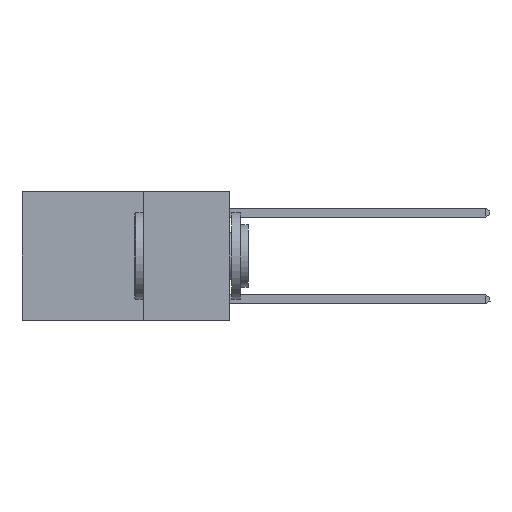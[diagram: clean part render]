
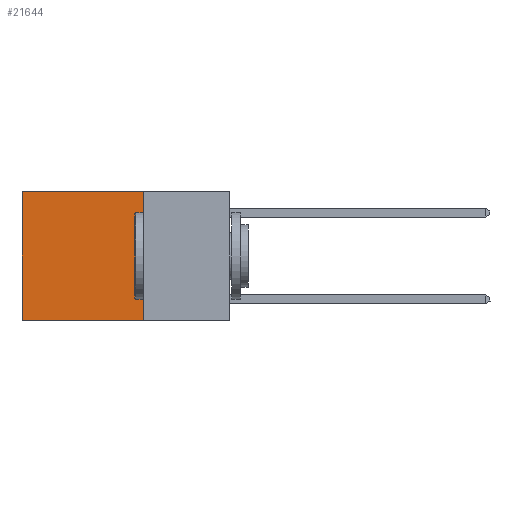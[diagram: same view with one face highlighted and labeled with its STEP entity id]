
A CAD part, left-side view. The second image highlights one B-rep face of the part: STEP entity #21644.
In plain terms, the highlighted planar face has unit normal (-1, 0, 0).
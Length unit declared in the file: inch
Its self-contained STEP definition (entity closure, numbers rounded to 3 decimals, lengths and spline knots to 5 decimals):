
#991 = CARTESIAN_POINT ( 'NONE',  ( 0.2625, 0.6, -0.37 ) ) ;
#1272 = VECTOR ( 'NONE', #6204, 39.37008 ) ;
#1865 = VECTOR ( 'NONE', #13802, 39.37008 ) ;
#3233 = VECTOR ( 'NONE', #29305, 39.37008 ) ;
#3928 = ORIENTED_EDGE ( 'NONE', *, *, #29902, .F. ) ;
#4036 = CARTESIAN_POINT ( 'NONE',  ( 0.2625, 0.25, -0.37 ) ) ;
#4430 = EDGE_CURVE ( 'NONE', #24362, #11835, #11613, .T. ) ;
#4773 = DIRECTION ( 'NONE',  ( 1., 0., 0. ) ) ;
#4872 = EDGE_CURVE ( 'NONE', #10754, #11835, #27289, .T. ) ;
#6083 = DIRECTION ( 'NONE',  ( 0., 1., 0. ) ) ;
#6204 = DIRECTION ( 'NONE',  ( 0., 1., 0. ) ) ;
#6263 = CARTESIAN_POINT ( 'NONE',  ( 0.2625, 0.25, -0.37 ) ) ;
#7657 = FACE_OUTER_BOUND ( 'NONE', #17735, .T. ) ;
#7757 = EDGE_CURVE ( 'NONE', #18770, #24362, #8125, .T. ) ;
#8125 = LINE ( 'NONE', #25061, #1272 ) ;
#10754 = VERTEX_POINT ( 'NONE', #6263 ) ;
#10882 = CARTESIAN_POINT ( 'NONE',  ( 0.2625, 0.6, 0. ) ) ;
#11613 = LINE ( 'NONE', #17572, #3233 ) ;
#11675 = CARTESIAN_POINT ( 'NONE',  ( 0.2625, 0.25, 0. ) ) ;
#11835 = VERTEX_POINT ( 'NONE', #991 ) ;
#13802 = DIRECTION ( 'NONE',  ( 0., 0., -1. ) ) ;
#14512 = ORIENTED_EDGE ( 'NONE', *, *, #4430, .T. ) ;
#16401 = AXIS2_PLACEMENT_3D ( 'NONE', #11675, #4773, #21297 ) ;
#17572 = CARTESIAN_POINT ( 'NONE',  ( 0.2625, 0.6, 0. ) ) ;
#17735 = EDGE_LOOP ( 'NONE', ( #14512, #29069, #3928, #19036 ) ) ;
#17902 = CARTESIAN_POINT ( 'NONE',  ( 0.2625, 0.25, 0. ) ) ;
#18770 = VERTEX_POINT ( 'NONE', #19895 ) ;
#19036 = ORIENTED_EDGE ( 'NONE', *, *, #7757, .T. ) ;
#19895 = CARTESIAN_POINT ( 'NONE',  ( 0.2625, 0.25, 0. ) ) ;
#21297 = DIRECTION ( 'NONE',  ( 0., 0., -1. ) ) ;
#21538 = LINE ( 'NONE', #17902, #1865 ) ;
#21644 = ADVANCED_FACE ( 'NONE', ( #7657 ), #25761, .F. ) ;
#24362 = VERTEX_POINT ( 'NONE', #10882 ) ;
#25061 = CARTESIAN_POINT ( 'NONE',  ( 0.2625, 0.25, 0. ) ) ;
#25761 = PLANE ( 'NONE',  #16401 ) ;
#26924 = VECTOR ( 'NONE', #6083, 39.37008 ) ;
#27289 = LINE ( 'NONE', #4036, #26924 ) ;
#29069 = ORIENTED_EDGE ( 'NONE', *, *, #4872, .F. ) ;
#29305 = DIRECTION ( 'NONE',  ( 0., 0., -1. ) ) ;
#29902 = EDGE_CURVE ( 'NONE', #18770, #10754, #21538, .T. ) ;
